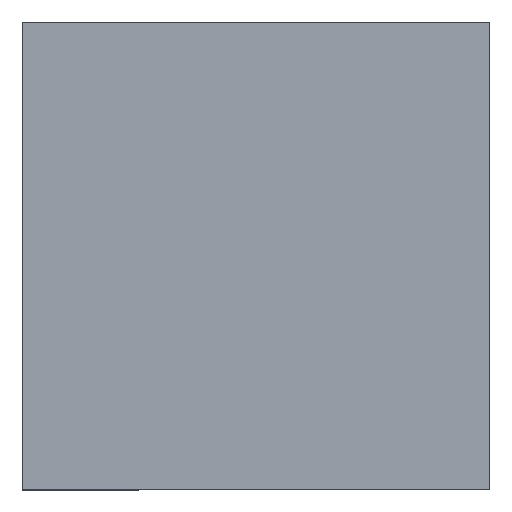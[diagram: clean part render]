
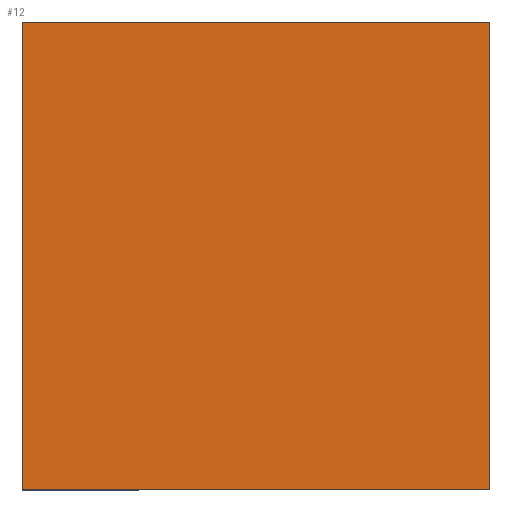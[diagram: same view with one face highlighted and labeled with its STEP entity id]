
A CAD part, top view. The second image highlights one B-rep face of the part: STEP entity #12.
In plain terms, the highlighted planar face has unit normal (0, 0, 1).
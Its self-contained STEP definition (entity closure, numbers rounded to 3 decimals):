
#10 = EDGE_CURVE ( 'NONE', #167, #26, #202, .T. ) ;
#12 = ADVANCED_FACE ( 'NONE', ( #152 ), #47, .F. ) ;
#13 = VECTOR ( 'NONE', #109, 1000. ) ;
#25 = DIRECTION ( 'NONE',  ( 0., 0., -1. ) ) ;
#26 = VERTEX_POINT ( 'NONE', #96 ) ;
#27 = CARTESIAN_POINT ( 'NONE',  ( -22.811, 20.5, 22.127 ) ) ;
#39 = ORIENTED_EDGE ( 'NONE', *, *, #10, .T. ) ;
#40 = CARTESIAN_POINT ( 'NONE',  ( -22.811, 20.5, 22.127 ) ) ;
#44 = CARTESIAN_POINT ( 'NONE',  ( 17.189, -19.5, 22.127 ) ) ;
#46 = ORIENTED_EDGE ( 'NONE', *, *, #193, .T. ) ;
#47 = PLANE ( 'NONE',  #172 ) ;
#51 = LINE ( 'NONE', #113, #63 ) ;
#52 = LINE ( 'NONE', #99, #13 ) ;
#53 = VECTOR ( 'NONE', #102, 1000. ) ;
#54 = VECTOR ( 'NONE', #83, 1000. ) ;
#59 = ORIENTED_EDGE ( 'NONE', *, *, #181, .T. ) ;
#63 = VECTOR ( 'NONE', #116, 1000. ) ;
#70 = CARTESIAN_POINT ( 'NONE',  ( 17.189, 20.5, 22.127 ) ) ;
#83 = DIRECTION ( 'NONE',  ( 0., -1., 0. ) ) ;
#85 = CARTESIAN_POINT ( 'NONE',  ( 0., 22.127, 22.127 ) ) ;
#87 = DIRECTION ( 'NONE',  ( 0., 1., 0. ) ) ;
#96 = CARTESIAN_POINT ( 'NONE',  ( -22.811, -19.5, 22.127 ) ) ;
#99 = CARTESIAN_POINT ( 'NONE',  ( -22.811, 20.5, 22.127 ) ) ;
#102 = DIRECTION ( 'NONE',  ( 0., 1., 0. ) ) ;
#105 = CARTESIAN_POINT ( 'NONE',  ( 17.189, 20.5, 22.127 ) ) ;
#109 = DIRECTION ( 'NONE',  ( -1., 0., 0. ) ) ;
#113 = CARTESIAN_POINT ( 'NONE',  ( -22.811, -19.5, 22.127 ) ) ;
#116 = DIRECTION ( 'NONE',  ( 1., 0., 0. ) ) ;
#117 = LINE ( 'NONE', #70, #53 ) ;
#122 = VERTEX_POINT ( 'NONE', #105 ) ;
#125 = VERTEX_POINT ( 'NONE', #44 ) ;
#128 = ORIENTED_EDGE ( 'NONE', *, *, #191, .T. ) ;
#152 = FACE_OUTER_BOUND ( 'NONE', #166, .T. ) ;
#166 = EDGE_LOOP ( 'NONE', ( #59, #39, #46, #128 ) ) ;
#167 = VERTEX_POINT ( 'NONE', #40 ) ;
#172 = AXIS2_PLACEMENT_3D ( 'NONE', #85, #25, #87 ) ;
#181 = EDGE_CURVE ( 'NONE', #122, #167, #52, .T. ) ;
#191 = EDGE_CURVE ( 'NONE', #125, #122, #117, .T. ) ;
#193 = EDGE_CURVE ( 'NONE', #26, #125, #51, .T. ) ;
#202 = LINE ( 'NONE', #27, #54 ) ;
